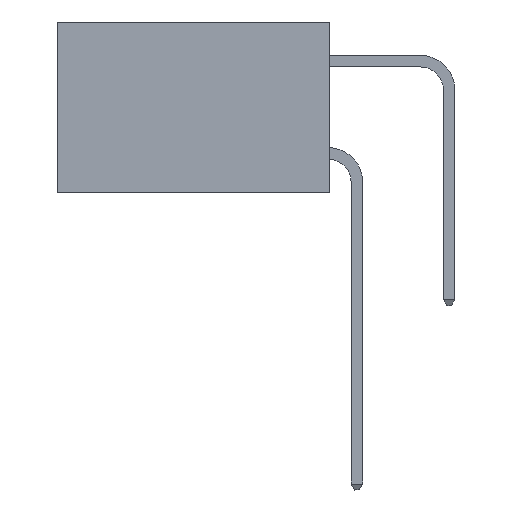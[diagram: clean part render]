
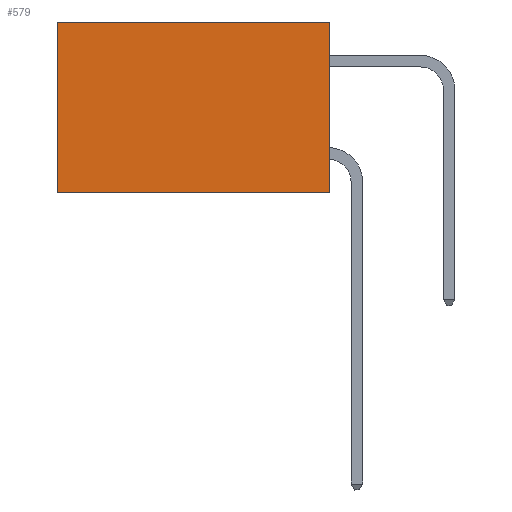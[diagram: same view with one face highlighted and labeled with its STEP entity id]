
A CAD part, left-side view. The second image highlights one B-rep face of the part: STEP entity #579.
In plain terms, the highlighted planar face has unit normal (-1, 0, 0).
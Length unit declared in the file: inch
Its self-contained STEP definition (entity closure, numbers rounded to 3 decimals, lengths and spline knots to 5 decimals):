
#579 = ADVANCED_FACE ( 'NONE', ( #8393 ), #23969, .F. ) ;
#657 = DIRECTION ( 'NONE',  ( 0., 0., -1. ) ) ;
#1656 = VECTOR ( 'NONE', #11260, 39.37008 ) ;
#3241 = EDGE_CURVE ( 'NONE', #16628, #22395, #21291, .T. ) ;
#3244 = LINE ( 'NONE', #10275, #15582 ) ;
#4098 = CARTESIAN_POINT ( 'NONE',  ( 0.277, 0., 0. ) ) ;
#5869 = AXIS2_PLACEMENT_3D ( 'NONE', #28755, #16705, #657 ) ;
#7413 = LINE ( 'NONE', #25272, #25444 ) ;
#8320 = EDGE_CURVE ( 'NONE', #16628, #23521, #3244, .T. ) ;
#8393 = FACE_OUTER_BOUND ( 'NONE', #15104, .T. ) ;
#9763 = CARTESIAN_POINT ( 'NONE',  ( 0.277, 0.59, -0.37 ) ) ;
#10275 = CARTESIAN_POINT ( 'NONE',  ( 0.277, 0., -0.37 ) ) ;
#11260 = DIRECTION ( 'NONE',  ( 0., 1., 0. ) ) ;
#11331 = ORIENTED_EDGE ( 'NONE', *, *, #17881, .F. ) ;
#11440 = ORIENTED_EDGE ( 'NONE', *, *, #3241, .T. ) ;
#12491 = CARTESIAN_POINT ( 'NONE',  ( 0.277, 0.59, -0.37 ) ) ;
#12768 = DIRECTION ( 'NONE',  ( 0., 0., -1. ) ) ;
#13456 = EDGE_CURVE ( 'NONE', #22395, #29784, #15758, .T. ) ;
#14976 = VECTOR ( 'NONE', #29481, 39.37008 ) ;
#15104 = EDGE_LOOP ( 'NONE', ( #15891, #11331, #15275, #11440 ) ) ;
#15212 = CARTESIAN_POINT ( 'NONE',  ( 0.277, 0.59, 0. ) ) ;
#15275 = ORIENTED_EDGE ( 'NONE', *, *, #8320, .F. ) ;
#15582 = VECTOR ( 'NONE', #12768, 39.37008 ) ;
#15758 = LINE ( 'NONE', #12491, #14976 ) ;
#15891 = ORIENTED_EDGE ( 'NONE', *, *, #13456, .T. ) ;
#16628 = VERTEX_POINT ( 'NONE', #4098 ) ;
#16705 = DIRECTION ( 'NONE',  ( 1., 0., 0. ) ) ;
#17881 = EDGE_CURVE ( 'NONE', #23521, #29784, #7413, .T. ) ;
#18036 = DIRECTION ( 'NONE',  ( 0., 1., 0. ) ) ;
#21291 = LINE ( 'NONE', #30520, #1656 ) ;
#22395 = VERTEX_POINT ( 'NONE', #15212 ) ;
#23521 = VERTEX_POINT ( 'NONE', #23831 ) ;
#23831 = CARTESIAN_POINT ( 'NONE',  ( 0.277, 0., -0.37 ) ) ;
#23969 = PLANE ( 'NONE',  #5869 ) ;
#25272 = CARTESIAN_POINT ( 'NONE',  ( 0.277, 0., -0.37 ) ) ;
#25444 = VECTOR ( 'NONE', #18036, 39.37008 ) ;
#28755 = CARTESIAN_POINT ( 'NONE',  ( 0.277, 0., -0.37 ) ) ;
#29481 = DIRECTION ( 'NONE',  ( 0., 0., -1. ) ) ;
#29784 = VERTEX_POINT ( 'NONE', #9763 ) ;
#30520 = CARTESIAN_POINT ( 'NONE',  ( 0.277, 0., 0. ) ) ;
